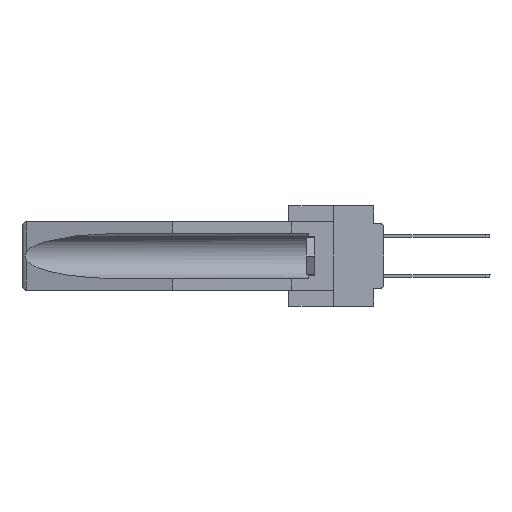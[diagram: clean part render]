
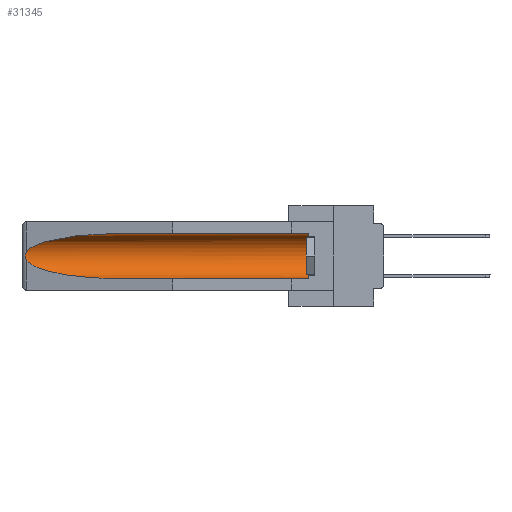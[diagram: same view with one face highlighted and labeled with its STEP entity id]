
A CAD part, left-side view. The second image highlights one B-rep face of the part: STEP entity #31345.
In plain terms, the highlighted cylindrical face has radius 2.857 mm (diameter 5.715 mm), a partial arc.
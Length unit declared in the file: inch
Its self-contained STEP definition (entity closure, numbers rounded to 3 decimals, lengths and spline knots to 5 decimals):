
#72 = EDGE_CURVE ( 'NONE', #4252, #2590, #380, .T. ) ;
#144 = CARTESIAN_POINT ( 'NONE',  ( 0.26654, 1.53092, -0.15636 ) ) ;
#380 = LINE ( 'NONE', #30867, #10270 ) ;
#560 =( BOUNDED_CURVE ( )  B_SPLINE_CURVE ( 3, ( #15983, #2992, #30792, #7995 ),
 .UNSPECIFIED., .F., .F. ) 
 B_SPLINE_CURVE_WITH_KNOTS ( ( 4, 4 ),
 ( 0.1948, 1.5708 ),
 .UNSPECIFIED. ) 
 CURVE ( )  GEOMETRIC_REPRESENTATION_ITEM ( )  RATIONAL_B_SPLINE_CURVE ( ( 1., 0.848, 0.848, 1. ) ) 
 REPRESENTATION_ITEM ( '' )  );
#920 = CARTESIAN_POINT ( 'NONE',  ( 0.26655, 1.53094, -0.18657 ) ) ;
#976 =( BOUNDED_CURVE ( )  B_SPLINE_CURVE ( 3, ( #25278, #32752, #2308, #22721 ),
 .UNSPECIFIED., .F., .F. ) 
 B_SPLINE_CURVE_WITH_KNOTS ( ( 4, 4 ),
 ( 4.71239, 6.08839 ),
 .UNSPECIFIED. ) 
 CURVE ( )  GEOMETRIC_REPRESENTATION_ITEM ( )  RATIONAL_B_SPLINE_CURVE ( ( 1., 0.848, 0.848, 1. ) ) 
 REPRESENTATION_ITEM ( '' )  );
#1315 = DIRECTION ( 'NONE',  ( 0., -1., 0. ) ) ;
#2308 = CARTESIAN_POINT ( 'NONE',  ( 0.25451, 1.48313, -0.09465 ) ) ;
#2590 = VERTEX_POINT ( 'NONE', #22823 ) ;
#2918 = EDGE_LOOP ( 'NONE', ( #25186, #18150, #5879, #25666, #27885, #29212 ) ) ;
#2992 = CARTESIAN_POINT ( 'NONE',  ( 0.25451, 1.48313, -0.24835 ) ) ;
#3055 = CARTESIAN_POINT ( 'NONE',  ( 0.155, -0.30754, -0.059 ) ) ;
#4252 = VERTEX_POINT ( 'NONE', #29988 ) ;
#4816 = CIRCLE ( 'NONE', #24288, 0.1125 ) ;
#5879 = ORIENTED_EDGE ( 'NONE', *, *, #16706, .T. ) ;
#7008 = CARTESIAN_POINT ( 'NONE',  ( 0.155, 0.126, -0.059 ) ) ;
#7995 = CARTESIAN_POINT ( 'NONE',  ( 0.155, 1.07973, -0.284 ) ) ;
#8215 = CARTESIAN_POINT ( 'NONE',  ( 0.2675, 1.53308, -0.17534 ) ) ;
#8536 = CARTESIAN_POINT ( 'NONE',  ( 0.26537, 1.52718, -0.19328 ) ) ;
#10270 = VECTOR ( 'NONE', #21408, 39.37008 ) ;
#10756 = CARTESIAN_POINT ( 'NONE',  ( 0.2673, 1.5327, -0.16383 ) ) ;
#11961 = FACE_OUTER_BOUND ( 'NONE', #2918, .T. ) ;
#12885 = DIRECTION ( 'NONE',  ( 0., 0., 1. ) ) ;
#13257 = EDGE_CURVE ( 'NONE', #21989, #28029, #976, .T. ) ;
#13417 = CARTESIAN_POINT ( 'NONE',  ( 0.26537, 1.52718, -0.19328 ) ) ;
#13787 = EDGE_CURVE ( 'NONE', #21031, #21989, #27492, .T. ) ;
#13996 = EDGE_CURVE ( 'NONE', #4252, #21031, #4816, .T. ) ;
#15018 = EDGE_CURVE ( 'NONE', #28029, #16859, #21094, .T. ) ;
#15983 = CARTESIAN_POINT ( 'NONE',  ( 0.26537, 1.52718, -0.19328 ) ) ;
#16706 = EDGE_CURVE ( 'NONE', #16859, #2590, #560, .T. ) ;
#16859 = VERTEX_POINT ( 'NONE', #8536 ) ;
#17848 = CARTESIAN_POINT ( 'NONE',  ( 0.26537, 1.52718, -0.14972 ) ) ;
#17914 = CYLINDRICAL_SURFACE ( 'NONE', #22109, 0.1125 ) ;
#18150 = ORIENTED_EDGE ( 'NONE', *, *, #15018, .T. ) ;
#19159 = CARTESIAN_POINT ( 'NONE',  ( 0.155, 1.07973, -0.059 ) ) ;
#21031 = VERTEX_POINT ( 'NONE', #7008 ) ;
#21087 = CARTESIAN_POINT ( 'NONE',  ( 0.2675, 1.53308, -0.16763 ) ) ;
#21094 = B_SPLINE_CURVE_WITH_KNOTS ( 'NONE', 3,
 ( #17848, #28012, #144, #10756, #21087, #8215, #28684, #920, #23531, #13417 ),
 .UNSPECIFIED., .F., .F.,
 ( 4, 2, 2, 2, 4 ),
 ( 0., 0.00029, 0.00058, 0.00087, 0.00117 ),
 .UNSPECIFIED. ) ;
#21268 = CARTESIAN_POINT ( 'NONE',  ( 0.155, 0.126, -0.1715 ) ) ;
#21408 = DIRECTION ( 'NONE',  ( 0., 1., 0. ) ) ;
#21989 = VERTEX_POINT ( 'NONE', #19159 ) ;
#22109 = AXIS2_PLACEMENT_3D ( 'NONE', #30371, #28374, #12885 ) ;
#22721 = CARTESIAN_POINT ( 'NONE',  ( 0.26537, 1.52718, -0.14972 ) ) ;
#22823 = CARTESIAN_POINT ( 'NONE',  ( 0.155, 1.07973, -0.284 ) ) ;
#23369 = DIRECTION ( 'NONE',  ( 0., 1., 0. ) ) ;
#23480 = VECTOR ( 'NONE', #23369, 39.37008 ) ;
#23531 = CARTESIAN_POINT ( 'NONE',  ( 0.26597, 1.5296, -0.19026 ) ) ;
#24288 = AXIS2_PLACEMENT_3D ( 'NONE', #21268, #1315, #29086 ) ;
#24936 = CARTESIAN_POINT ( 'NONE',  ( 0.26537, 1.52718, -0.14972 ) ) ;
#25186 = ORIENTED_EDGE ( 'NONE', *, *, #13257, .T. ) ;
#25278 = CARTESIAN_POINT ( 'NONE',  ( 0.155, 1.07973, -0.059 ) ) ;
#25666 = ORIENTED_EDGE ( 'NONE', *, *, #72, .F. ) ;
#27492 = LINE ( 'NONE', #3055, #23480 ) ;
#27885 = ORIENTED_EDGE ( 'NONE', *, *, #13996, .T. ) ;
#28012 = CARTESIAN_POINT ( 'NONE',  ( 0.26597, 1.52961, -0.15275 ) ) ;
#28029 = VERTEX_POINT ( 'NONE', #24936 ) ;
#28374 = DIRECTION ( 'NONE',  ( 0., 1., 0. ) ) ;
#28684 = CARTESIAN_POINT ( 'NONE',  ( 0.2673, 1.53269, -0.17917 ) ) ;
#29086 = DIRECTION ( 'NONE',  ( 0., 0., 1. ) ) ;
#29212 = ORIENTED_EDGE ( 'NONE', *, *, #13787, .T. ) ;
#29988 = CARTESIAN_POINT ( 'NONE',  ( 0.155, 0.126, -0.284 ) ) ;
#30371 = CARTESIAN_POINT ( 'NONE',  ( 0.155, -0.30754, -0.1715 ) ) ;
#30792 = CARTESIAN_POINT ( 'NONE',  ( 0.21114, 1.30732, -0.284 ) ) ;
#30867 = CARTESIAN_POINT ( 'NONE',  ( 0.155, -0.30754, -0.284 ) ) ;
#31345 = ADVANCED_FACE ( 'NONE', ( #11961 ), #17914, .F. ) ;
#32752 = CARTESIAN_POINT ( 'NONE',  ( 0.21114, 1.30732, -0.059 ) ) ;
